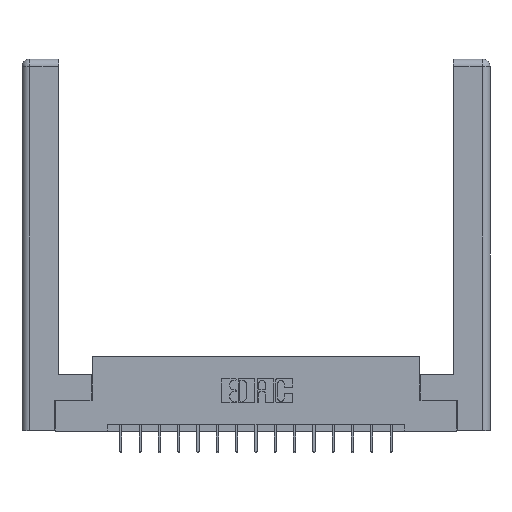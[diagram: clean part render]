
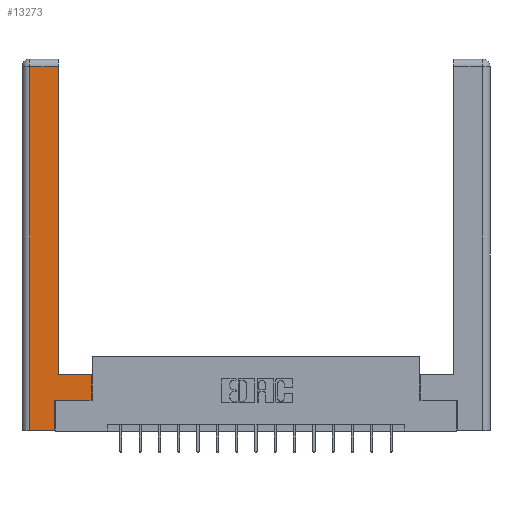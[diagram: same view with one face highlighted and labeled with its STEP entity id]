
A CAD part, top view. The second image highlights one B-rep face of the part: STEP entity #13273.
In plain terms, the highlighted planar face has unit normal (0, 0, 1).
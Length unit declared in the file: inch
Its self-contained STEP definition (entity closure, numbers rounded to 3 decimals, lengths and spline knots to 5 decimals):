
#14 = CARTESIAN_POINT ( 'NONE',  ( 0.295, 0.45, 0. ) ) ;
#152 = VECTOR ( 'NONE', #11206, 39.37008 ) ;
#317 = CARTESIAN_POINT ( 'NONE',  ( 0.0615, 2.94, 0. ) ) ;
#379 = CARTESIAN_POINT ( 'NONE',  ( 0.565, 0.45, 0. ) ) ;
#412 = VECTOR ( 'NONE', #12616, 39.37008 ) ;
#438 = DIRECTION ( 'NONE',  ( 0., 1., 0. ) ) ;
#502 = CARTESIAN_POINT ( 'NONE',  ( 0.565, 0.245, 0. ) ) ;
#729 = VECTOR ( 'NONE', #8137, 39.37008 ) ;
#777 = VECTOR ( 'NONE', #16858, 39.37008 ) ;
#1203 = LINE ( 'NONE', #4788, #2455 ) ;
#1385 = CARTESIAN_POINT ( 'NONE',  ( 0.565, 0.45, 0. ) ) ;
#1475 = CARTESIAN_POINT ( 'NONE',  ( 0.295, 2.94, 0. ) ) ;
#1936 = EDGE_CURVE ( 'NONE', #5424, #9290, #7492, .T. ) ;
#2217 = LINE ( 'NONE', #2631, #729 ) ;
#2237 = VECTOR ( 'NONE', #438, 39.37008 ) ;
#2437 = VERTEX_POINT ( 'NONE', #1475 ) ;
#2444 = EDGE_CURVE ( 'NONE', #2437, #17125, #11134, .T. ) ;
#2455 = VECTOR ( 'NONE', #14450, 39.37008 ) ;
#2631 = CARTESIAN_POINT ( 'NONE',  ( 0.265, 0.245, 0. ) ) ;
#2903 = ORIENTED_EDGE ( 'NONE', *, *, #4335, .T. ) ;
#2949 = ORIENTED_EDGE ( 'NONE', *, *, #15350, .T. ) ;
#2970 = VERTEX_POINT ( 'NONE', #4948 ) ;
#4048 = EDGE_CURVE ( 'NONE', #10679, #10076, #1203, .T. ) ;
#4294 = CARTESIAN_POINT ( 'NONE',  ( 0.265, 0., 0. ) ) ;
#4335 = EDGE_CURVE ( 'NONE', #9290, #2437, #17152, .T. ) ;
#4469 = CARTESIAN_POINT ( 'NONE',  ( 0.295, 3., 0. ) ) ;
#4788 = CARTESIAN_POINT ( 'NONE',  ( 0.265, 0., 0. ) ) ;
#4809 = EDGE_CURVE ( 'NONE', #2970, #5424, #16720, .T. ) ;
#4948 = CARTESIAN_POINT ( 'NONE',  ( 0.565, 0.245, 0. ) ) ;
#5038 = AXIS2_PLACEMENT_3D ( 'NONE', #5585, #12434, #9710 ) ;
#5261 = ORIENTED_EDGE ( 'NONE', *, *, #12147, .T. ) ;
#5424 = VERTEX_POINT ( 'NONE', #1385 ) ;
#5585 = CARTESIAN_POINT ( 'NONE',  ( 0., 0., 0. ) ) ;
#6331 = EDGE_CURVE ( 'NONE', #9596, #2970, #10577, .T. ) ;
#6760 = ORIENTED_EDGE ( 'NONE', *, *, #6331, .T. ) ;
#7492 = LINE ( 'NONE', #12438, #412 ) ;
#8137 = DIRECTION ( 'NONE',  ( 0., 1., 0. ) ) ;
#8596 = CARTESIAN_POINT ( 'NONE',  ( 0.0615, 0., 0. ) ) ;
#8782 = CARTESIAN_POINT ( 'NONE',  ( 0.0615, 2.94, 0. ) ) ;
#9290 = VERTEX_POINT ( 'NONE', #14 ) ;
#9596 = VERTEX_POINT ( 'NONE', #11939 ) ;
#9710 = DIRECTION ( 'NONE',  ( -1., 0., 0. ) ) ;
#10076 = VERTEX_POINT ( 'NONE', #4294 ) ;
#10577 = LINE ( 'NONE', #502, #11662 ) ;
#10679 = VERTEX_POINT ( 'NONE', #8596 ) ;
#11134 = LINE ( 'NONE', #317, #152 ) ;
#11206 = DIRECTION ( 'NONE',  ( -1., 0., 0. ) ) ;
#11662 = VECTOR ( 'NONE', #14160, 39.37008 ) ;
#11677 = DIRECTION ( 'NONE',  ( 0., -1., 0. ) ) ;
#11939 = CARTESIAN_POINT ( 'NONE',  ( 0.265, 0.245, 0. ) ) ;
#12147 = EDGE_CURVE ( 'NONE', #17125, #10679, #14593, .T. ) ;
#12434 = DIRECTION ( 'NONE',  ( 0., 0., -1. ) ) ;
#12438 = CARTESIAN_POINT ( 'NONE',  ( 0.295, 0.45, 0. ) ) ;
#12446 = ORIENTED_EDGE ( 'NONE', *, *, #2444, .T. ) ;
#12616 = DIRECTION ( 'NONE',  ( -1., 0., 0. ) ) ;
#12860 = VECTOR ( 'NONE', #11677, 39.37008 ) ;
#13273 = ADVANCED_FACE ( 'NONE', ( #17793 ), #13812, .F. ) ;
#13812 = PLANE ( 'NONE',  #5038 ) ;
#13900 = ORIENTED_EDGE ( 'NONE', *, *, #4809, .T. ) ;
#14160 = DIRECTION ( 'NONE',  ( 1., 0., 0. ) ) ;
#14450 = DIRECTION ( 'NONE',  ( 1., 0., 0. ) ) ;
#14582 = ORIENTED_EDGE ( 'NONE', *, *, #1936, .T. ) ;
#14593 = LINE ( 'NONE', #15913, #12860 ) ;
#15350 = EDGE_CURVE ( 'NONE', #10076, #9596, #2217, .T. ) ;
#15635 = ORIENTED_EDGE ( 'NONE', *, *, #4048, .T. ) ;
#15913 = CARTESIAN_POINT ( 'NONE',  ( 0.0615, 0., 0. ) ) ;
#16005 = EDGE_LOOP ( 'NONE', ( #2903, #12446, #5261, #15635, #2949, #6760, #13900, #14582 ) ) ;
#16720 = LINE ( 'NONE', #379, #2237 ) ;
#16858 = DIRECTION ( 'NONE',  ( 0., 1., 0. ) ) ;
#17125 = VERTEX_POINT ( 'NONE', #8782 ) ;
#17152 = LINE ( 'NONE', #4469, #777 ) ;
#17793 = FACE_OUTER_BOUND ( 'NONE', #16005, .T. ) ;
